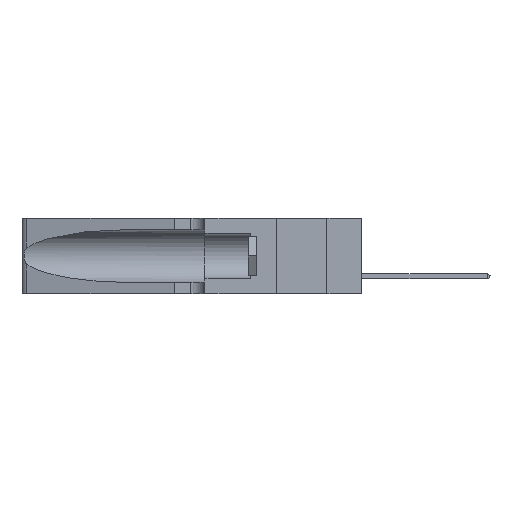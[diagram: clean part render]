
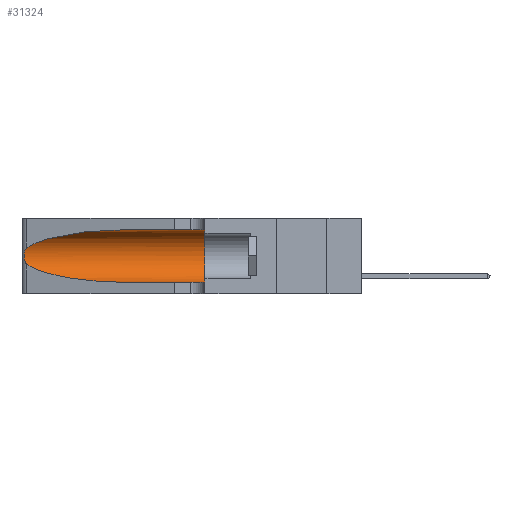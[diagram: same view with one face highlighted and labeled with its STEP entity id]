
A CAD part, left-side view. The second image highlights one B-rep face of the part: STEP entity #31324.
In plain terms, the highlighted cylindrical face has radius 3.308 mm (diameter 6.617 mm), a partial arc.
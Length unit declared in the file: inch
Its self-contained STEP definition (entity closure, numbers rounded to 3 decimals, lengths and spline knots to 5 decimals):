
#1033 = CIRCLE ( 'NONE', #38607, 0.13025 ) ;
#1302 = CARTESIAN_POINT ( 'NONE',  ( 0.25854, 1.2359, 0.20912 ) ) ;
#1368 = ORIENTED_EDGE ( 'NONE', *, *, #6030, .T. ) ;
#2370 = DIRECTION ( 'NONE',  ( 0., -1., 0. ) ) ;
#2511 = ORIENTED_EDGE ( 'NONE', *, *, #24575, .T. ) ;
#2678 = VERTEX_POINT ( 'NONE', #25110 ) ;
#2837 = CARTESIAN_POINT ( 'NONE',  ( 0.1305, 0.35, 0.05475 ) ) ;
#3420 =( BOUNDED_CURVE ( )  B_SPLINE_CURVE ( 3, ( #28310, #4624, #4467, #7640 ),
 .UNSPECIFIED., .F., .F. ) 
 B_SPLINE_CURVE_WITH_KNOTS ( ( 4, 4 ),
 ( 1.5708, 2.84003 ),
 .UNSPECIFIED. ) 
 CURVE ( )  GEOMETRIC_REPRESENTATION_ITEM ( )  RATIONAL_B_SPLINE_CURVE ( ( 1., 0.87, 0.87, 1. ) ) 
 REPRESENTATION_ITEM ( '' )  );
#4074 = CARTESIAN_POINT ( 'NONE',  ( 0.25856, 1.23593, 0.16098 ) ) ;
#4246 = CARTESIAN_POINT ( 'NONE',  ( 0.25487, 1.22718, 0.22369 ) ) ;
#4467 = CARTESIAN_POINT ( 'NONE',  ( 0.2373, 1.15595, 0.28018 ) ) ;
#4578 = DIRECTION ( 'NONE',  ( 0., 1., 0. ) ) ;
#4624 = CARTESIAN_POINT ( 'NONE',  ( 0.18966, 0.96281, 0.31525 ) ) ;
#6022 = LINE ( 'NONE', #19827, #24231 ) ;
#6030 = EDGE_CURVE ( 'NONE', #35396, #30837, #33682, .T. ) ;
#7107 = CARTESIAN_POINT ( 'NONE',  ( 0.25639, 1.23186, 0.15144 ) ) ;
#7640 = CARTESIAN_POINT ( 'NONE',  ( 0.25487, 1.22718, 0.22369 ) ) ;
#8312 = CARTESIAN_POINT ( 'NONE',  ( 0.1305, 1.61858, 0.05475 ) ) ;
#10123 = CARTESIAN_POINT ( 'NONE',  ( 0.25487, 1.22718, 0.14631 ) ) ;
#10465 = CARTESIAN_POINT ( 'NONE',  ( 0.1305, 0.35, 0.185 ) ) ;
#11117 = LINE ( 'NONE', #8312, #14449 ) ;
#11765 = CARTESIAN_POINT ( 'NONE',  ( 0.2373, 1.15595, 0.08982 ) ) ;
#12768 = CARTESIAN_POINT ( 'NONE',  ( 0.1305, 1.61858, 0.185 ) ) ;
#13279 = CARTESIAN_POINT ( 'NONE',  ( 0.25487, 1.22718, 0.22369 ) ) ;
#14089 = ORIENTED_EDGE ( 'NONE', *, *, #24203, .T. ) ;
#14449 = VECTOR ( 'NONE', #2370, 39.37008 ) ;
#16022 = CARTESIAN_POINT ( 'NONE',  ( 0.26075, 1.23896, 0.19203 ) ) ;
#17953 = CARTESIAN_POINT ( 'NONE',  ( 0.25487, 1.22718, 0.14631 ) ) ;
#19040 = CARTESIAN_POINT ( 'NONE',  ( 0.26075, 1.23896, 0.178 ) ) ;
#19359 = ORIENTED_EDGE ( 'NONE', *, *, #32612, .F. ) ;
#19827 = CARTESIAN_POINT ( 'NONE',  ( 0.1305, 1.61858, 0.31525 ) ) ;
#19943 = CARTESIAN_POINT ( 'NONE',  ( 0.1305, 0.72297, 0.05475 ) ) ;
#21050 = CARTESIAN_POINT ( 'NONE',  ( 0.25487, 1.22718, 0.14631 ) ) ;
#21988 = ORIENTED_EDGE ( 'NONE', *, *, #33637, .T. ) ;
#22314 = CARTESIAN_POINT ( 'NONE',  ( 0.26017, 1.23833, 0.17102 ) ) ;
#22499 = FACE_OUTER_BOUND ( 'NONE', #36313, .T. ) ;
#22596 = DIRECTION ( 'NONE',  ( 0., 0., -1. ) ) ;
#22670 = ORIENTED_EDGE ( 'NONE', *, *, #24041, .F. ) ;
#22758 = VERTEX_POINT ( 'NONE', #27522 ) ;
#23229 = VERTEX_POINT ( 'NONE', #4246 ) ;
#24041 = EDGE_CURVE ( 'NONE', #22758, #2678, #6022, .T. ) ;
#24203 = EDGE_CURVE ( 'NONE', #22758, #23229, #3420, .T. ) ;
#24231 = VECTOR ( 'NONE', #37475, 39.37008 ) ;
#24575 = EDGE_CURVE ( 'NONE', #30837, #32876, #11117, .T. ) ;
#25035 = CARTESIAN_POINT ( 'NONE',  ( 0.25789, 1.23486, 0.15765 ) ) ;
#25110 = CARTESIAN_POINT ( 'NONE',  ( 0.1305, 0.35, 0.31525 ) ) ;
#25241 = DIRECTION ( 'NONE',  ( 0., 0., 1. ) ) ;
#27522 = CARTESIAN_POINT ( 'NONE',  ( 0.1305, 0.72297, 0.31525 ) ) ;
#28065 = CARTESIAN_POINT ( 'NONE',  ( 0.25555, 1.22993, 0.14849 ) ) ;
#28310 = CARTESIAN_POINT ( 'NONE',  ( 0.1305, 0.72297, 0.31525 ) ) ;
#28438 = B_SPLINE_CURVE_WITH_KNOTS ( 'NONE', 3,
 ( #13279, #33286, #36315, #34222, #1302, #33945, #16022, #19040, #22314, #4074, #25035, #7107, #28065, #10123 ),
 .UNSPECIFIED., .F., .F.,
 ( 4, 2, 2, 2, 2, 2, 4 ),
 ( 0., 0.00027, 0.00053, 0.00107, 0.0016, 0.00187, 0.00214 ),
 .UNSPECIFIED. ) ;
#28979 = AXIS2_PLACEMENT_3D ( 'NONE', #12768, #33819, #22596 ) ;
#29827 = CARTESIAN_POINT ( 'NONE',  ( 0.18966, 0.96281, 0.05475 ) ) ;
#30837 = VERTEX_POINT ( 'NONE', #19943 ) ;
#31324 = ADVANCED_FACE ( 'NONE', ( #22499 ), #31373, .F. ) ;
#31373 = CYLINDRICAL_SURFACE ( 'NONE', #28979, 0.13025 ) ;
#32612 = EDGE_CURVE ( 'NONE', #2678, #32876, #1033, .T. ) ;
#32706 = CARTESIAN_POINT ( 'NONE',  ( 0.1305, 0.72297, 0.05475 ) ) ;
#32876 = VERTEX_POINT ( 'NONE', #2837 ) ;
#33286 = CARTESIAN_POINT ( 'NONE',  ( 0.25555, 1.22994, 0.2215 ) ) ;
#33637 = EDGE_CURVE ( 'NONE', #23229, #35396, #28438, .T. ) ;
#33682 =( BOUNDED_CURVE ( )  B_SPLINE_CURVE ( 3, ( #17953, #11765, #29827, #32706 ),
 .UNSPECIFIED., .F., .F. ) 
 B_SPLINE_CURVE_WITH_KNOTS ( ( 4, 4 ),
 ( 3.44316, 4.71239 ),
 .UNSPECIFIED. ) 
 CURVE ( )  GEOMETRIC_REPRESENTATION_ITEM ( )  RATIONAL_B_SPLINE_CURVE ( ( 1., 0.87, 0.87, 1. ) ) 
 REPRESENTATION_ITEM ( '' )  );
#33819 = DIRECTION ( 'NONE',  ( 0., -1., 0. ) ) ;
#33945 = CARTESIAN_POINT ( 'NONE',  ( 0.26018, 1.23835, 0.19895 ) ) ;
#34222 = CARTESIAN_POINT ( 'NONE',  ( 0.25787, 1.23484, 0.2124 ) ) ;
#35396 = VERTEX_POINT ( 'NONE', #21050 ) ;
#36313 = EDGE_LOOP ( 'NONE', ( #14089, #21988, #1368, #2511, #19359, #22670 ) ) ;
#36315 = CARTESIAN_POINT ( 'NONE',  ( 0.25639, 1.23184, 0.21858 ) ) ;
#37475 = DIRECTION ( 'NONE',  ( 0., -1., 0. ) ) ;
#38607 = AXIS2_PLACEMENT_3D ( 'NONE', #10465, #4578, #25241 ) ;
